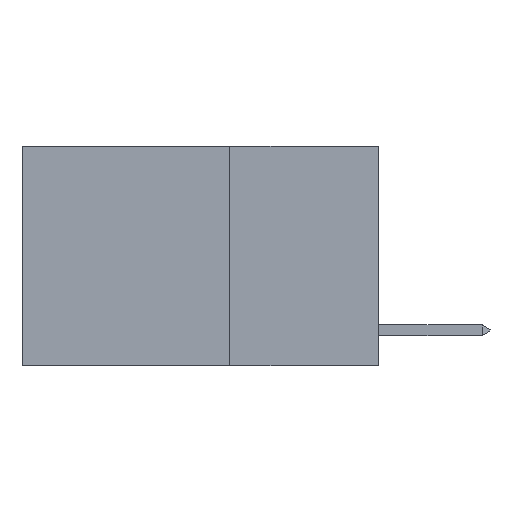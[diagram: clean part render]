
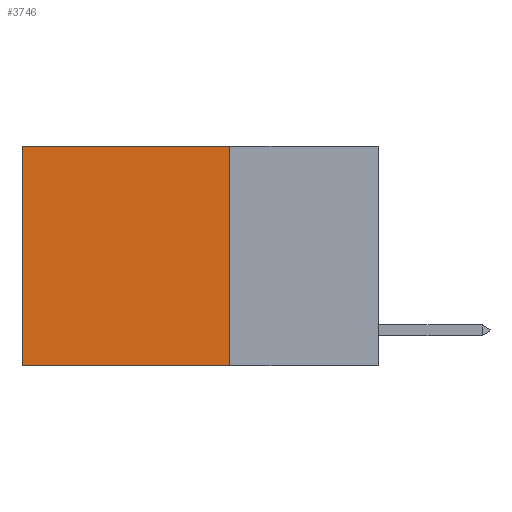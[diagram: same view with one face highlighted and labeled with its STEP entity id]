
A CAD part, left-side view. The second image highlights one B-rep face of the part: STEP entity #3746.
In plain terms, the highlighted planar face has unit normal (-1, 0, 0).
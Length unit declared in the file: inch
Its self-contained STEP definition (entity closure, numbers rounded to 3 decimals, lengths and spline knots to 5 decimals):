
#751 = VECTOR ( 'NONE', #6608, 39.37008 ) ;
#1068 = VECTOR ( 'NONE', #9417, 39.37008 ) ;
#1565 = LINE ( 'NONE', #9375, #1068 ) ;
#1923 = EDGE_CURVE ( 'NONE', #14339, #7458, #1565, .T. ) ;
#2210 = EDGE_CURVE ( 'NONE', #15632, #7458, #6784, .T. ) ;
#3146 = VECTOR ( 'NONE', #16198, 39.37008 ) ;
#3672 = LINE ( 'NONE', #3836, #3146 ) ;
#3746 = ADVANCED_FACE ( 'NONE', ( #5748 ), #9171, .F. ) ;
#3836 = CARTESIAN_POINT ( 'NONE',  ( 0.2625, 0.25, 0. ) ) ;
#5748 = FACE_OUTER_BOUND ( 'NONE', #9026, .T. ) ;
#6608 = DIRECTION ( 'NONE',  ( 0., 0., -1. ) ) ;
#6784 = LINE ( 'NONE', #17267, #14440 ) ;
#7458 = VERTEX_POINT ( 'NONE', #8864 ) ;
#8864 = CARTESIAN_POINT ( 'NONE',  ( 0.2625, 0.6, -0.37 ) ) ;
#8984 = DIRECTION ( 'NONE',  ( 0., 0., -1. ) ) ;
#9026 = EDGE_LOOP ( 'NONE', ( #10705, #17959, #16013, #10925 ) ) ;
#9036 = DIRECTION ( 'NONE',  ( 1., 0., 0. ) ) ;
#9062 = CARTESIAN_POINT ( 'NONE',  ( 0.2625, 0.25, 0. ) ) ;
#9171 = PLANE ( 'NONE',  #17465 ) ;
#9375 = CARTESIAN_POINT ( 'NONE',  ( 0.2625, 0.25, -0.37 ) ) ;
#9417 = DIRECTION ( 'NONE',  ( 0., 1., 0. ) ) ;
#10541 = VERTEX_POINT ( 'NONE', #11739 ) ;
#10705 = ORIENTED_EDGE ( 'NONE', *, *, #2210, .T. ) ;
#10925 = ORIENTED_EDGE ( 'NONE', *, *, #15881, .T. ) ;
#11739 = CARTESIAN_POINT ( 'NONE',  ( 0.2625, 0.25, 0. ) ) ;
#12301 = LINE ( 'NONE', #15708, #751 ) ;
#14112 = CARTESIAN_POINT ( 'NONE',  ( 0.2625, 0.6, 0. ) ) ;
#14296 = EDGE_CURVE ( 'NONE', #10541, #14339, #12301, .T. ) ;
#14305 = CARTESIAN_POINT ( 'NONE',  ( 0.2625, 0.25, -0.37 ) ) ;
#14339 = VERTEX_POINT ( 'NONE', #14305 ) ;
#14440 = VECTOR ( 'NONE', #17093, 39.37008 ) ;
#15632 = VERTEX_POINT ( 'NONE', #14112 ) ;
#15708 = CARTESIAN_POINT ( 'NONE',  ( 0.2625, 0.25, 0. ) ) ;
#15881 = EDGE_CURVE ( 'NONE', #10541, #15632, #3672, .T. ) ;
#16013 = ORIENTED_EDGE ( 'NONE', *, *, #14296, .F. ) ;
#16198 = DIRECTION ( 'NONE',  ( 0., 1., 0. ) ) ;
#17093 = DIRECTION ( 'NONE',  ( 0., 0., -1. ) ) ;
#17267 = CARTESIAN_POINT ( 'NONE',  ( 0.2625, 0.6, 0. ) ) ;
#17465 = AXIS2_PLACEMENT_3D ( 'NONE', #9062, #9036, #8984 ) ;
#17959 = ORIENTED_EDGE ( 'NONE', *, *, #1923, .F. ) ;
